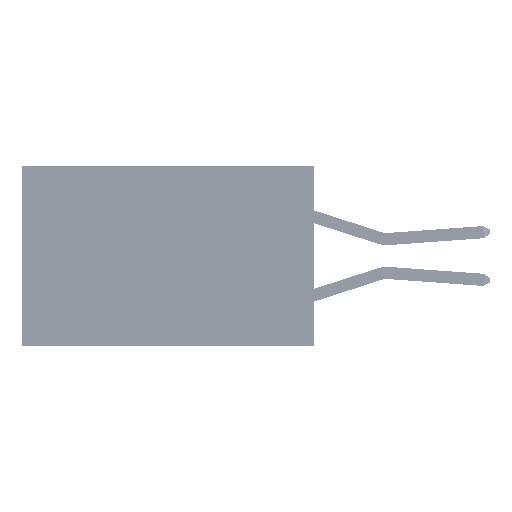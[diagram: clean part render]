
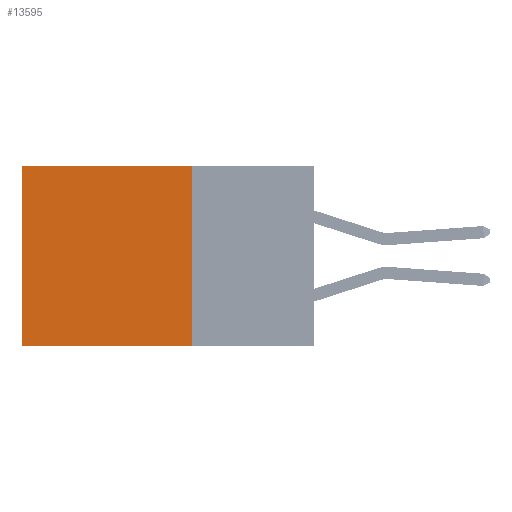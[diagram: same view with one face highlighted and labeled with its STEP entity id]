
A CAD part, left-side view. The second image highlights one B-rep face of the part: STEP entity #13595.
In plain terms, the highlighted planar face has unit normal (-1, 0, 0).
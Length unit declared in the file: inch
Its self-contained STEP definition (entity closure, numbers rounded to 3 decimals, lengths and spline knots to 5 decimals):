
#620 = VECTOR ( 'NONE', #12285, 39.37008 ) ;
#2430 = VECTOR ( 'NONE', #20454, 39.37008 ) ;
#3683 = PLANE ( 'NONE',  #36525 ) ;
#4423 = LINE ( 'NONE', #4473, #620 ) ;
#4473 = CARTESIAN_POINT ( 'NONE',  ( 0.2875, 0.25, 0. ) ) ;
#5543 = DIRECTION ( 'NONE',  ( 0., 1., 0. ) ) ;
#7614 = DIRECTION ( 'NONE',  ( 1., 0., 0. ) ) ;
#8129 = DIRECTION ( 'NONE',  ( 0., 0., -1. ) ) ;
#9336 = EDGE_CURVE ( 'NONE', #28670, #35959, #46109, .T. ) ;
#10794 = ORIENTED_EDGE ( 'NONE', *, *, #35596, .T. ) ;
#11271 = CARTESIAN_POINT ( 'NONE',  ( 0.2875, 0.25, 0. ) ) ;
#12033 = CARTESIAN_POINT ( 'NONE',  ( 0.2875, 0.25, 0. ) ) ;
#12285 = DIRECTION ( 'NONE',  ( 0., 1., 0. ) ) ;
#13210 = ORIENTED_EDGE ( 'NONE', *, *, #9336, .T. ) ;
#13595 = ADVANCED_FACE ( 'NONE', ( #17809 ), #3683, .F. ) ;
#17306 = EDGE_CURVE ( 'NONE', #44972, #47402, #19297, .T. ) ;
#17809 = FACE_OUTER_BOUND ( 'NONE', #25797, .T. ) ;
#19297 = LINE ( 'NONE', #20082, #21221 ) ;
#20082 = CARTESIAN_POINT ( 'NONE',  ( 0.2875, 0.25, 0. ) ) ;
#20454 = DIRECTION ( 'NONE',  ( 0., 0., -1. ) ) ;
#21221 = VECTOR ( 'NONE', #25011, 39.37008 ) ;
#25011 = DIRECTION ( 'NONE',  ( 0., 0., -1. ) ) ;
#25553 = CARTESIAN_POINT ( 'NONE',  ( 0.2875, 0.25, -0.37 ) ) ;
#25797 = EDGE_LOOP ( 'NONE', ( #13210, #42606, #34472, #10794 ) ) ;
#26760 = CARTESIAN_POINT ( 'NONE',  ( 0.2875, 0.6, -0.37 ) ) ;
#28445 = LINE ( 'NONE', #25553, #42957 ) ;
#28670 = VERTEX_POINT ( 'NONE', #39751 ) ;
#28937 = CARTESIAN_POINT ( 'NONE',  ( 0.2875, 0.6, 0. ) ) ;
#34472 = ORIENTED_EDGE ( 'NONE', *, *, #17306, .F. ) ;
#35596 = EDGE_CURVE ( 'NONE', #44972, #28670, #4423, .T. ) ;
#35959 = VERTEX_POINT ( 'NONE', #26760 ) ;
#36525 = AXIS2_PLACEMENT_3D ( 'NONE', #12033, #7614, #8129 ) ;
#39751 = CARTESIAN_POINT ( 'NONE',  ( 0.2875, 0.6, 0. ) ) ;
#42100 = CARTESIAN_POINT ( 'NONE',  ( 0.2875, 0.25, -0.37 ) ) ;
#42606 = ORIENTED_EDGE ( 'NONE', *, *, #42652, .F. ) ;
#42652 = EDGE_CURVE ( 'NONE', #47402, #35959, #28445, .T. ) ;
#42957 = VECTOR ( 'NONE', #5543, 39.37008 ) ;
#44972 = VERTEX_POINT ( 'NONE', #11271 ) ;
#46109 = LINE ( 'NONE', #28937, #2430 ) ;
#47402 = VERTEX_POINT ( 'NONE', #42100 ) ;
